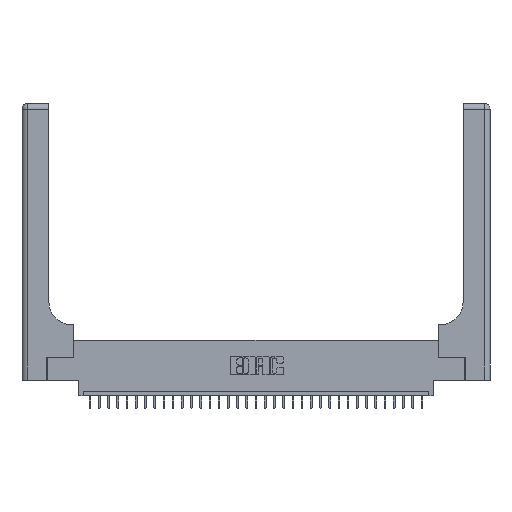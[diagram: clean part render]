
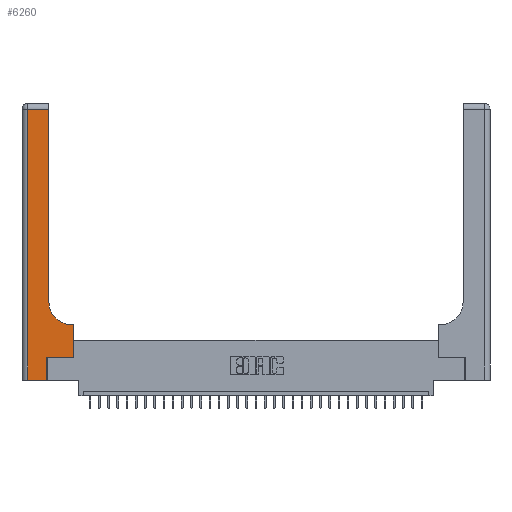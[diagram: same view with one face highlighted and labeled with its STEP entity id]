
A CAD part, top view. The second image highlights one B-rep face of the part: STEP entity #6260.
In plain terms, the highlighted planar face has unit normal (0, 0, 1).
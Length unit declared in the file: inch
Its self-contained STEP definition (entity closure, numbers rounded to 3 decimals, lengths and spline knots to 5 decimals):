
#236 = LINE ( 'NONE', #29854, #8008 ) ;
#481 = CARTESIAN_POINT ( 'NONE',  ( 0.06, 2.94, 0.37 ) ) ;
#727 = DIRECTION ( 'NONE',  ( -1., 0., 0. ) ) ;
#1403 = CARTESIAN_POINT ( 'NONE',  ( 0.2915, 0.85, 0.37 ) ) ;
#1550 = CARTESIAN_POINT ( 'NONE',  ( 0.5585, 0.25, 0.37 ) ) ;
#1607 = EDGE_CURVE ( 'NONE', #16070, #33395, #32279, .T. ) ;
#2984 = DIRECTION ( 'NONE',  ( 1., 0., 0. ) ) ;
#3123 = ORIENTED_EDGE ( 'NONE', *, *, #23715, .T. ) ;
#3204 = ORIENTED_EDGE ( 'NONE', *, *, #15119, .T. ) ;
#3325 = VECTOR ( 'NONE', #22892, 39.37008 ) ;
#3881 = EDGE_LOOP ( 'NONE', ( #7923, #3204, #14460, #22471, #14452, #30228, #32115, #3123, #27922 ) ) ;
#4246 = EDGE_CURVE ( 'NONE', #25796, #6105, #29251, .T. ) ;
#4599 = CARTESIAN_POINT ( 'NONE',  ( 0.269, 0.25, 0.37 ) ) ;
#5383 = DIRECTION ( 'NONE',  ( 1., 0., 0. ) ) ;
#5518 = CARTESIAN_POINT ( 'NONE',  ( 0.5585, 0.6, 0.37 ) ) ;
#6053 = CARTESIAN_POINT ( 'NONE',  ( 0., 0., 0.37 ) ) ;
#6105 = VERTEX_POINT ( 'NONE', #6916 ) ;
#6226 = LINE ( 'NONE', #6053, #29561 ) ;
#6260 = ADVANCED_FACE ( 'NONE', ( #26610 ), #8774, .F. ) ;
#6405 = DIRECTION ( 'NONE',  ( 1., 0., 0. ) ) ;
#6538 = DIRECTION ( 'NONE',  ( 0., 1., 0. ) ) ;
#6916 = CARTESIAN_POINT ( 'NONE',  ( 0.06, 0., 0.37 ) ) ;
#7923 = ORIENTED_EDGE ( 'NONE', *, *, #1607, .T. ) ;
#8008 = VECTOR ( 'NONE', #2984, 39.37008 ) ;
#8154 = CARTESIAN_POINT ( 'NONE',  ( 0.06, 3., 0.37 ) ) ;
#8774 = PLANE ( 'NONE',  #26472 ) ;
#8958 = DIRECTION ( 'NONE',  ( 0., 1., 0. ) ) ;
#9195 = EDGE_CURVE ( 'NONE', #10162, #9285, #236, .T. ) ;
#9285 = VERTEX_POINT ( 'NONE', #1550 ) ;
#9344 = DIRECTION ( 'NONE',  ( -1., 0., 0. ) ) ;
#9633 = VERTEX_POINT ( 'NONE', #29307 ) ;
#9686 = CARTESIAN_POINT ( 'NONE',  ( 0., 2.94, 0.37 ) ) ;
#10162 = VERTEX_POINT ( 'NONE', #4599 ) ;
#11070 = CARTESIAN_POINT ( 'NONE',  ( 0.269, 0., 0.37 ) ) ;
#12315 = VECTOR ( 'NONE', #13291, 39.37008 ) ;
#12575 = AXIS2_PLACEMENT_3D ( 'NONE', #23542, #28887, #5383 ) ;
#13291 = DIRECTION ( 'NONE',  ( 0., -1., 0. ) ) ;
#14452 = ORIENTED_EDGE ( 'NONE', *, *, #31723, .T. ) ;
#14460 = ORIENTED_EDGE ( 'NONE', *, *, #4246, .T. ) ;
#15119 = EDGE_CURVE ( 'NONE', #33395, #25796, #29659, .T. ) ;
#15190 = LINE ( 'NONE', #20999, #3325 ) ;
#15817 = CARTESIAN_POINT ( 'NONE',  ( 0.2915, 2.94, 0.37 ) ) ;
#15976 = CARTESIAN_POINT ( 'NONE',  ( 0., 3., 0.37 ) ) ;
#16070 = VERTEX_POINT ( 'NONE', #1403 ) ;
#16196 = LINE ( 'NONE', #11070, #32964 ) ;
#18028 = VECTOR ( 'NONE', #27881, 39.37008 ) ;
#19023 = CARTESIAN_POINT ( 'NONE',  ( 0.2915, 3., 0.37 ) ) ;
#19445 = VERTEX_POINT ( 'NONE', #5518 ) ;
#20999 = CARTESIAN_POINT ( 'NONE',  ( 0.5585, 0.25, 0.37 ) ) ;
#21460 = CARTESIAN_POINT ( 'NONE',  ( 0.269, 0., 0.37 ) ) ;
#22471 = ORIENTED_EDGE ( 'NONE', *, *, #33593, .T. ) ;
#22892 = DIRECTION ( 'NONE',  ( 0., 1., 0. ) ) ;
#22958 = CIRCLE ( 'NONE', #12575, 0.25 ) ;
#23026 = LINE ( 'NONE', #27862, #23326 ) ;
#23326 = VECTOR ( 'NONE', #9344, 39.37008 ) ;
#23542 = CARTESIAN_POINT ( 'NONE',  ( 0.5415, 0.85, 0.37 ) ) ;
#23715 = EDGE_CURVE ( 'NONE', #19445, #9633, #23026, .T. ) ;
#24363 = DIRECTION ( 'NONE',  ( 0., 0., -1. ) ) ;
#25796 = VERTEX_POINT ( 'NONE', #481 ) ;
#26472 = AXIS2_PLACEMENT_3D ( 'NONE', #15976, #24363, #727 ) ;
#26610 = FACE_OUTER_BOUND ( 'NONE', #3881, .T. ) ;
#27640 = VERTEX_POINT ( 'NONE', #21460 ) ;
#27862 = CARTESIAN_POINT ( 'NONE',  ( 0.2915, 0.6, 0.37 ) ) ;
#27881 = DIRECTION ( 'NONE',  ( -1., 0., 0. ) ) ;
#27922 = ORIENTED_EDGE ( 'NONE', *, *, #33185, .T. ) ;
#28725 = VECTOR ( 'NONE', #6538, 39.37008 ) ;
#28858 = EDGE_CURVE ( 'NONE', #9285, #19445, #15190, .T. ) ;
#28887 = DIRECTION ( 'NONE',  ( 0., 0., -1. ) ) ;
#29251 = LINE ( 'NONE', #8154, #12315 ) ;
#29307 = CARTESIAN_POINT ( 'NONE',  ( 0.5415, 0.6, 0.37 ) ) ;
#29561 = VECTOR ( 'NONE', #6405, 39.37008 ) ;
#29659 = LINE ( 'NONE', #9686, #18028 ) ;
#29854 = CARTESIAN_POINT ( 'NONE',  ( 0.269, 0.25, 0.37 ) ) ;
#30228 = ORIENTED_EDGE ( 'NONE', *, *, #9195, .T. ) ;
#31723 = EDGE_CURVE ( 'NONE', #27640, #10162, #16196, .T. ) ;
#32115 = ORIENTED_EDGE ( 'NONE', *, *, #28858, .T. ) ;
#32279 = LINE ( 'NONE', #19023, #28725 ) ;
#32964 = VECTOR ( 'NONE', #8958, 39.37008 ) ;
#33185 = EDGE_CURVE ( 'NONE', #9633, #16070, #22958, .T. ) ;
#33395 = VERTEX_POINT ( 'NONE', #15817 ) ;
#33593 = EDGE_CURVE ( 'NONE', #6105, #27640, #6226, .T. ) ;
